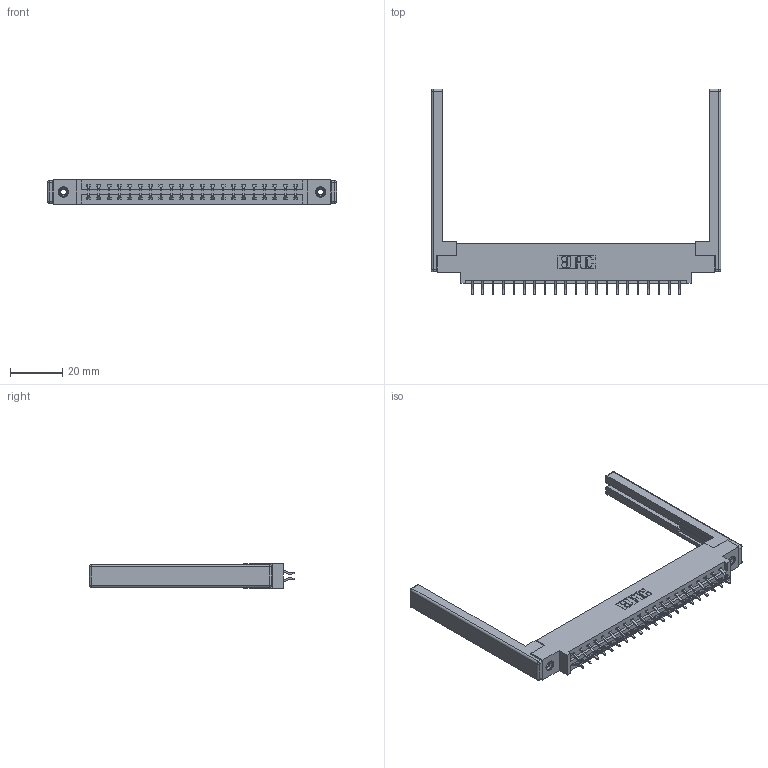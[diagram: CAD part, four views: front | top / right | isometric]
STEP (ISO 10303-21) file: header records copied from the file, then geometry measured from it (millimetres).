
FILE_DESCRIPTION (( 'STEP AP203' ), '1' );
FILE_NAME ('387-042-556-868.STEP', '2019-10-18T04:41:24', ( '' ), ( '' ), 'SwSTEP 2.0', 'SolidWorks 2016', '' );
FILE_SCHEMA (( 'CONFIG_CONTROL_DESIGN' ));
Length unit declared in the file: inch
Products named in the file (5): 337 Part_0.170 Offset - 0.156 Dia-TI; 387-042-556-868; 307-220-068; 345-292-001_556 Tail; 345-250-001_345-250-001-102
Assembly tree (47 placements, depth 2):
  387-042-556-868
    337 Part_0.170 Offset - 0.156 Dia-TI
    345-292-001_556 Tail  x42
    345-250-001_345-250-001-102  x2
    307-220-068  x2
Bounding box: 110.64 x 78.63 x 9.4 mm (x, y, z)
Volume: 15646.5 mm3; surface area: 16625.2 mm2
Topology: 47 solids, 47 shells, 2792 faces, 8231 edges, 5410 vertices
Faces by surface type: plane 1926, cylinder 842, cone 12, sphere 8, torus 4
Entity records: 22110 total; most frequent: CARTESIAN_POINT 3723, ORIENTED_EDGE 3636, DIRECTION 3264, EDGE_CURVE 1818, LINE 1632, VECTOR 1632, VERTEX_POINT 1202, AXIS2_PLACEMENT_3D 816
